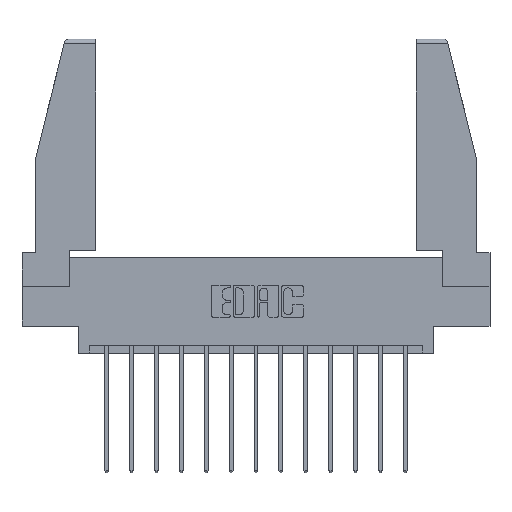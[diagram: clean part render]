
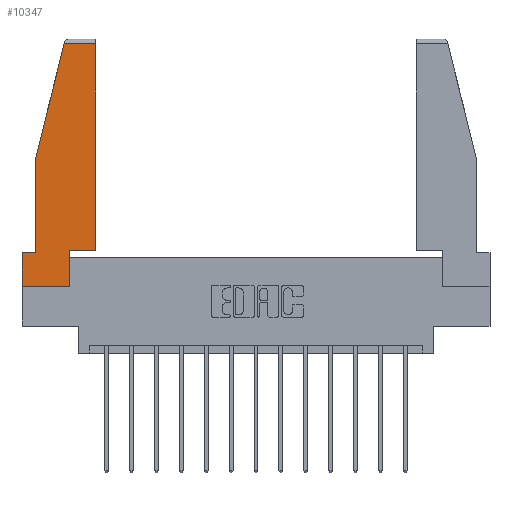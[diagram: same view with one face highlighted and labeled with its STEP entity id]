
A CAD part, top view. The second image highlights one B-rep face of the part: STEP entity #10347.
In plain terms, the highlighted planar face has unit normal (0, 0, 1).
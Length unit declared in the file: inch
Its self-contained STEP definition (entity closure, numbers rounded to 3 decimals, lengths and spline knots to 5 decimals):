
#132 = FACE_OUTER_BOUND ( 'NONE', #2349, .T. ) ;
#506 = LINE ( 'NONE', #11441, #7905 ) ;
#509 = DIRECTION ( 'NONE',  ( 0., -1., 0. ) ) ;
#1363 = DIRECTION ( 'NONE',  ( 1., 0., 0. ) ) ;
#1383 = DIRECTION ( 'NONE',  ( 1., 0., 0. ) ) ;
#1748 = ORIENTED_EDGE ( 'NONE', *, *, #9426, .T. ) ;
#1820 = CARTESIAN_POINT ( 'NONE',  ( 0.297, 0.223, 0. ) ) ;
#1972 = LINE ( 'NONE', #16211, #11738 ) ;
#2053 = VECTOR ( 'NONE', #5108, 39.37008 ) ;
#2271 = LINE ( 'NONE', #5154, #2053 ) ;
#2349 = EDGE_LOOP ( 'NONE', ( #12644, #6807, #13694, #3000, #1748, #4481, #4813, #6084, #10206 ) ) ;
#2431 = CARTESIAN_POINT ( 'NONE',  ( 0., 0., 0. ) ) ;
#2488 = LINE ( 'NONE', #10257, #6682 ) ;
#2540 = VERTEX_POINT ( 'NONE', #10166 ) ;
#3000 = ORIENTED_EDGE ( 'NONE', *, *, #5423, .T. ) ;
#3120 = EDGE_CURVE ( 'NONE', #3258, #10778, #2488, .T. ) ;
#3258 = VERTEX_POINT ( 'NONE', #1820 ) ;
#3294 = EDGE_CURVE ( 'NONE', #4770, #10210, #2271, .T. ) ;
#3320 = AXIS2_PLACEMENT_3D ( 'NONE', #9028, #8967, #1363 ) ;
#3511 = EDGE_CURVE ( 'NONE', #5476, #4770, #14408, .T. ) ;
#4277 = CARTESIAN_POINT ( 'NONE',  ( 0., 1.52, 0. ) ) ;
#4481 = ORIENTED_EDGE ( 'NONE', *, *, #3511, .T. ) ;
#4682 = CARTESIAN_POINT ( 'NONE',  ( 0., 0.21, 0. ) ) ;
#4770 = VERTEX_POINT ( 'NONE', #2431 ) ;
#4813 = ORIENTED_EDGE ( 'NONE', *, *, #3294, .T. ) ;
#5102 = CARTESIAN_POINT ( 'NONE',  ( 0., 0.21, 0. ) ) ;
#5108 = DIRECTION ( 'NONE',  ( 1., 0., 0. ) ) ;
#5154 = CARTESIAN_POINT ( 'NONE',  ( 0., 0., 0. ) ) ;
#5423 = EDGE_CURVE ( 'NONE', #2540, #6217, #7021, .T. ) ;
#5476 = VERTEX_POINT ( 'NONE', #14046 ) ;
#6084 = ORIENTED_EDGE ( 'NONE', *, *, #7360, .T. ) ;
#6186 = CARTESIAN_POINT ( 'NONE',  ( 0.2636, 1.52, 0. ) ) ;
#6217 = VERTEX_POINT ( 'NONE', #10695 ) ;
#6682 = VECTOR ( 'NONE', #1383, 39.37008 ) ;
#6807 = ORIENTED_EDGE ( 'NONE', *, *, #8539, .T. ) ;
#7021 = LINE ( 'NONE', #13886, #11591 ) ;
#7100 = CARTESIAN_POINT ( 'NONE',  ( 0.461, 1.52, 0. ) ) ;
#7360 = EDGE_CURVE ( 'NONE', #10210, #3258, #1972, .T. ) ;
#7447 = DIRECTION ( 'NONE',  ( -1., 0., 0. ) ) ;
#7838 = CARTESIAN_POINT ( 'NONE',  ( 0.461, 0.223, 0. ) ) ;
#7856 = LINE ( 'NONE', #7838, #13169 ) ;
#7905 = VECTOR ( 'NONE', #14062, 39.37008 ) ;
#7965 = VECTOR ( 'NONE', #8145, 39.37008 ) ;
#8145 = DIRECTION ( 'NONE',  ( -1., 0., 0. ) ) ;
#8539 = EDGE_CURVE ( 'NONE', #9367, #15723, #12882, .T. ) ;
#8755 = CARTESIAN_POINT ( 'NONE',  ( 0.297, 0., 0. ) ) ;
#8797 = CARTESIAN_POINT ( 'NONE',  ( 0.461, 0.223, 0. ) ) ;
#8967 = DIRECTION ( 'NONE',  ( 0., 0., 1. ) ) ;
#9028 = CARTESIAN_POINT ( 'NONE',  ( 0., 0., 0. ) ) ;
#9367 = VERTEX_POINT ( 'NONE', #7100 ) ;
#9426 = EDGE_CURVE ( 'NONE', #6217, #5476, #10858, .T. ) ;
#10079 = VECTOR ( 'NONE', #7447, 39.37008 ) ;
#10166 = CARTESIAN_POINT ( 'NONE',  ( 0.086, 0.8, 0. ) ) ;
#10206 = ORIENTED_EDGE ( 'NONE', *, *, #3120, .T. ) ;
#10210 = VERTEX_POINT ( 'NONE', #8755 ) ;
#10257 = CARTESIAN_POINT ( 'NONE',  ( 0.297, 0.223, 0. ) ) ;
#10347 = ADVANCED_FACE ( 'NONE', ( #132 ), #14019, .T. ) ;
#10695 = CARTESIAN_POINT ( 'NONE',  ( 0.086, 0.21, 0. ) ) ;
#10778 = VERTEX_POINT ( 'NONE', #8797 ) ;
#10858 = LINE ( 'NONE', #4682, #10079 ) ;
#10887 = EDGE_CURVE ( 'NONE', #15723, #2540, #506, .T. ) ;
#11238 = VECTOR ( 'NONE', #509, 39.37008 ) ;
#11320 = DIRECTION ( 'NONE',  ( 0., -1., 0. ) ) ;
#11441 = CARTESIAN_POINT ( 'NONE',  ( 0.271, 1.55, 0. ) ) ;
#11591 = VECTOR ( 'NONE', #11320, 39.37008 ) ;
#11738 = VECTOR ( 'NONE', #13066, 39.37008 ) ;
#12068 = EDGE_CURVE ( 'NONE', #10778, #9367, #7856, .T. ) ;
#12644 = ORIENTED_EDGE ( 'NONE', *, *, #12068, .T. ) ;
#12882 = LINE ( 'NONE', #4277, #7965 ) ;
#13066 = DIRECTION ( 'NONE',  ( 0., 1., 0. ) ) ;
#13169 = VECTOR ( 'NONE', #14253, 39.37008 ) ;
#13694 = ORIENTED_EDGE ( 'NONE', *, *, #10887, .T. ) ;
#13886 = CARTESIAN_POINT ( 'NONE',  ( 0.086, 0.8, 0. ) ) ;
#14019 = PLANE ( 'NONE',  #3320 ) ;
#14046 = CARTESIAN_POINT ( 'NONE',  ( 0., 0.21, 0. ) ) ;
#14062 = DIRECTION ( 'NONE',  ( -0.239, -0.971, 0. ) ) ;
#14253 = DIRECTION ( 'NONE',  ( 0., 1., 0. ) ) ;
#14408 = LINE ( 'NONE', #5102, #11238 ) ;
#15723 = VERTEX_POINT ( 'NONE', #6186 ) ;
#16211 = CARTESIAN_POINT ( 'NONE',  ( 0.297, 0., 0. ) ) ;
